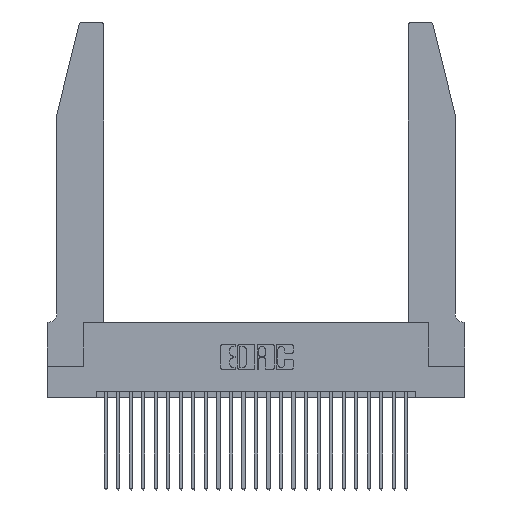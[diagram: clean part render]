
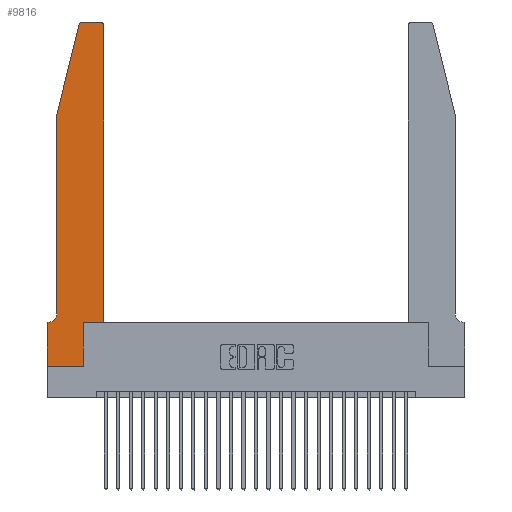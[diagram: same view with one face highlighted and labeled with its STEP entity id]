
A CAD part, top view. The second image highlights one B-rep face of the part: STEP entity #9816.
In plain terms, the highlighted planar face has unit normal (0, 0, 1).
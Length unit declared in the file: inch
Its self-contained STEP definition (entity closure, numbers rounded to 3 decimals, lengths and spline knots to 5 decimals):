
#18 = CIRCLE ( 'NONE', #25258, 0.03 ) ;
#146 = EDGE_CURVE ( 'NONE', #8877, #19762, #11343, .T. ) ;
#1601 = EDGE_CURVE ( 'NONE', #17807, #17557, #4316, .T. ) ;
#1713 = DIRECTION ( 'NONE',  ( 0., 1., 0. ) ) ;
#1965 = LINE ( 'NONE', #4662, #22553 ) ;
#2067 = CARTESIAN_POINT ( 'NONE',  ( 0.0755, 2., 0.37 ) ) ;
#2183 = VERTEX_POINT ( 'NONE', #11626 ) ;
#2482 = CARTESIAN_POINT ( 'NONE',  ( 0.25487, 2.72718, 0.37 ) ) ;
#2855 = CARTESIAN_POINT ( 'NONE',  ( 0.4505, 0.35, 0.37 ) ) ;
#2997 = VERTEX_POINT ( 'NONE', #24485 ) ;
#3401 = ORIENTED_EDGE ( 'NONE', *, *, #1601, .T. ) ;
#3467 = VERTEX_POINT ( 'NONE', #17082 ) ;
#3473 = ORIENTED_EDGE ( 'NONE', *, *, #24853, .T. ) ;
#3538 = ORIENTED_EDGE ( 'NONE', *, *, #146, .T. ) ;
#3543 = EDGE_CURVE ( 'NONE', #7054, #17807, #24561, .T. ) ;
#3867 = VECTOR ( 'NONE', #12192, 39.37008 ) ;
#4165 = CARTESIAN_POINT ( 'NONE',  ( 0.0755, 0.35, 0.37 ) ) ;
#4316 = LINE ( 'NONE', #24274, #25628 ) ;
#4318 = CARTESIAN_POINT ( 'NONE',  ( 0.2865, 0.35, 0.37 ) ) ;
#4515 = LINE ( 'NONE', #22461, #3867 ) ;
#4662 = CARTESIAN_POINT ( 'NONE',  ( 0.4505, 0.35, 0.37 ) ) ;
#5120 = LINE ( 'NONE', #19730, #15433 ) ;
#5212 = VECTOR ( 'NONE', #1713, 39.37008 ) ;
#5365 = CARTESIAN_POINT ( 'NONE',  ( 0., 0.35, 0.37 ) ) ;
#5798 = DIRECTION ( 'NONE',  ( 1., 0., 0. ) ) ;
#5913 = PLANE ( 'NONE',  #8548 ) ;
#6081 = CARTESIAN_POINT ( 'NONE',  ( 0.4205, 2.72, 0.37 ) ) ;
#6216 = DIRECTION ( 'NONE',  ( -1., 0., 0. ) ) ;
#6770 = VERTEX_POINT ( 'NONE', #22847 ) ;
#7054 = VERTEX_POINT ( 'NONE', #5365 ) ;
#7170 = LINE ( 'NONE', #4318, #13280 ) ;
#7291 = EDGE_CURVE ( 'NONE', #19762, #13677, #12052, .T. ) ;
#8005 = DIRECTION ( 'NONE',  ( 0., 0., 1. ) ) ;
#8145 = DIRECTION ( 'NONE',  ( 1., 0., 0. ) ) ;
#8257 = ORIENTED_EDGE ( 'NONE', *, *, #7291, .T. ) ;
#8548 = AXIS2_PLACEMENT_3D ( 'NONE', #20335, #8005, #22396 ) ;
#8712 = DIRECTION ( 'NONE',  ( 1., 0., 0. ) ) ;
#8877 = VERTEX_POINT ( 'NONE', #2855 ) ;
#8970 = VECTOR ( 'NONE', #10257, 39.37008 ) ;
#8981 = ORIENTED_EDGE ( 'NONE', *, *, #24141, .T. ) ;
#9041 = DIRECTION ( 'NONE',  ( 0., -1., 0. ) ) ;
#9506 = AXIS2_PLACEMENT_3D ( 'NONE', #6081, #20492, #8145 ) ;
#9510 = VERTEX_POINT ( 'NONE', #14927 ) ;
#9816 = ADVANCED_FACE ( 'NONE', ( #25487 ), #5913, .T. ) ;
#10219 = DIRECTION ( 'NONE',  ( 0., 0., -1. ) ) ;
#10257 = DIRECTION ( 'NONE',  ( 0., -1., 0. ) ) ;
#10765 = ORIENTED_EDGE ( 'NONE', *, *, #19019, .T. ) ;
#10981 = EDGE_CURVE ( 'NONE', #9510, #7054, #11568, .T. ) ;
#11343 = LINE ( 'NONE', #11954, #5212 ) ;
#11568 = LINE ( 'NONE', #4165, #21883 ) ;
#11626 = CARTESIAN_POINT ( 'NONE',  ( 0.0755, 2., 0.37 ) ) ;
#11745 = DIRECTION ( 'NONE',  ( 0., 0., 1. ) ) ;
#11954 = CARTESIAN_POINT ( 'NONE',  ( 0.4505, 0.35, 0.37 ) ) ;
#12016 = CARTESIAN_POINT ( 'NONE',  ( 0.2865, 0., 0.37 ) ) ;
#12052 = CIRCLE ( 'NONE', #9506, 0.03 ) ;
#12192 = DIRECTION ( 'NONE',  ( -1., 0., 0. ) ) ;
#12416 = ORIENTED_EDGE ( 'NONE', *, *, #19376, .T. ) ;
#13280 = VECTOR ( 'NONE', #20808, 39.37008 ) ;
#13561 = EDGE_CURVE ( 'NONE', #2183, #2997, #19281, .T. ) ;
#13677 = VERTEX_POINT ( 'NONE', #25054 ) ;
#14124 = EDGE_CURVE ( 'NONE', #2997, #9510, #16680, .T. ) ;
#14581 = ORIENTED_EDGE ( 'NONE', *, *, #10981, .T. ) ;
#14927 = CARTESIAN_POINT ( 'NONE',  ( 0.0055, 0.35, 0.37 ) ) ;
#15433 = VECTOR ( 'NONE', #19935, 39.37008 ) ;
#15537 = AXIS2_PLACEMENT_3D ( 'NONE', #22541, #10219, #24644 ) ;
#16680 = CIRCLE ( 'NONE', #15537, 0.07 ) ;
#17082 = CARTESIAN_POINT ( 'NONE',  ( 0.2865, 0.35, 0.37 ) ) ;
#17437 = ORIENTED_EDGE ( 'NONE', *, *, #13561, .T. ) ;
#17557 = VERTEX_POINT ( 'NONE', #12016 ) ;
#17807 = VERTEX_POINT ( 'NONE', #23451 ) ;
#19019 = EDGE_CURVE ( 'NONE', #3467, #8877, #1965, .T. ) ;
#19281 = LINE ( 'NONE', #2067, #8970 ) ;
#19376 = EDGE_CURVE ( 'NONE', #13677, #6770, #4515, .T. ) ;
#19730 = CARTESIAN_POINT ( 'NONE',  ( 0.0755, 2., 0.37 ) ) ;
#19762 = VERTEX_POINT ( 'NONE', #25834 ) ;
#19932 = ORIENTED_EDGE ( 'NONE', *, *, #14124, .T. ) ;
#19935 = DIRECTION ( 'NONE',  ( -0.239, -0.971, 0. ) ) ;
#20210 = EDGE_LOOP ( 'NONE', ( #12416, #8981, #3473, #17437, #19932, #14581, #22907, #3401, #20892, #10765, #3538, #8257 ) ) ;
#20335 = CARTESIAN_POINT ( 'NONE',  ( 0., 0.35, 0.37 ) ) ;
#20492 = DIRECTION ( 'NONE',  ( 0., 0., 1. ) ) ;
#20808 = DIRECTION ( 'NONE',  ( 0., 1., 0. ) ) ;
#20892 = ORIENTED_EDGE ( 'NONE', *, *, #21706, .T. ) ;
#21706 = EDGE_CURVE ( 'NONE', #17557, #3467, #7170, .T. ) ;
#21883 = VECTOR ( 'NONE', #6216, 39.37008 ) ;
#22396 = DIRECTION ( 'NONE',  ( 1., 0., 0. ) ) ;
#22461 = CARTESIAN_POINT ( 'NONE',  ( 0.2605, 2.75, 0.37 ) ) ;
#22541 = CARTESIAN_POINT ( 'NONE',  ( 0.0055, 0.42, 0.37 ) ) ;
#22553 = VECTOR ( 'NONE', #8712, 39.37008 ) ;
#22847 = CARTESIAN_POINT ( 'NONE',  ( 0.284, 2.75, 0.37 ) ) ;
#22907 = ORIENTED_EDGE ( 'NONE', *, *, #3543, .T. ) ;
#23243 = VECTOR ( 'NONE', #9041, 39.37008 ) ;
#23451 = CARTESIAN_POINT ( 'NONE',  ( 0., 0., 0.37 ) ) ;
#24108 = CARTESIAN_POINT ( 'NONE',  ( 0.284, 2.72, 0.37 ) ) ;
#24141 = EDGE_CURVE ( 'NONE', #6770, #26275, #18, .T. ) ;
#24274 = CARTESIAN_POINT ( 'NONE',  ( 0., 0., 0.37 ) ) ;
#24485 = CARTESIAN_POINT ( 'NONE',  ( 0.0755, 0.42, 0.37 ) ) ;
#24561 = LINE ( 'NONE', #25486, #23243 ) ;
#24644 = DIRECTION ( 'NONE',  ( -1., 0., 0. ) ) ;
#24853 = EDGE_CURVE ( 'NONE', #26275, #2183, #5120, .T. ) ;
#25054 = CARTESIAN_POINT ( 'NONE',  ( 0.4205, 2.75, 0.37 ) ) ;
#25258 = AXIS2_PLACEMENT_3D ( 'NONE', #24108, #11745, #26211 ) ;
#25486 = CARTESIAN_POINT ( 'NONE',  ( 0., 0., 0.37 ) ) ;
#25487 = FACE_OUTER_BOUND ( 'NONE', #20210, .T. ) ;
#25628 = VECTOR ( 'NONE', #5798, 39.37008 ) ;
#25834 = CARTESIAN_POINT ( 'NONE',  ( 0.4505, 2.72, 0.37 ) ) ;
#26211 = DIRECTION ( 'NONE',  ( 1., 0., 0. ) ) ;
#26275 = VERTEX_POINT ( 'NONE', #2482 ) ;
